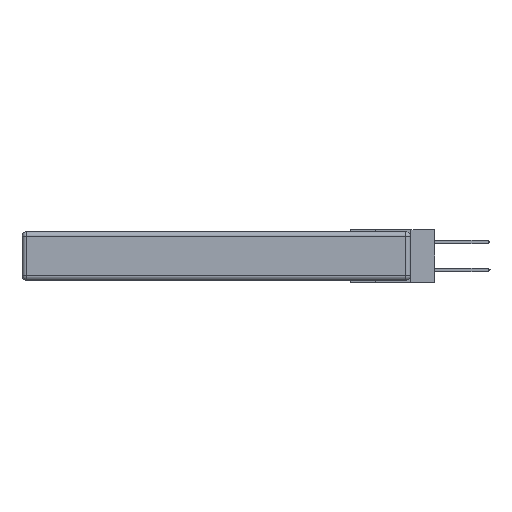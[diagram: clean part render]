
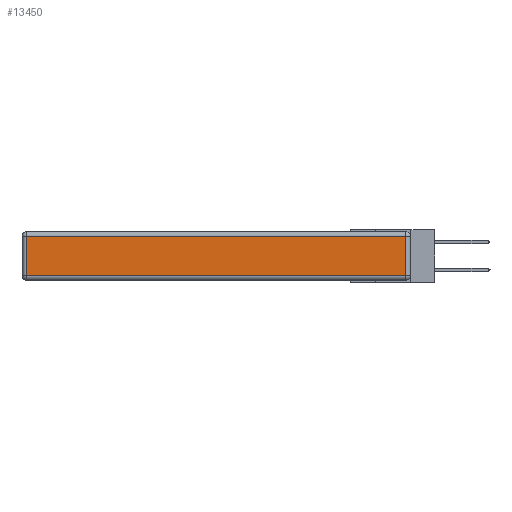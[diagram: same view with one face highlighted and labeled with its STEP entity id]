
A CAD part, left-side view. The second image highlights one B-rep face of the part: STEP entity #13450.
In plain terms, the highlighted planar face has unit normal (-1, 0, 0).
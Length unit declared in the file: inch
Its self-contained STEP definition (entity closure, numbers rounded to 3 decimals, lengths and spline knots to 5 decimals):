
#124 = CARTESIAN_POINT ( 'NONE',  ( 0., 0., -0.343 ) ) ;
#168 = DIRECTION ( 'NONE',  ( -1., 0., 0. ) ) ;
#174 = EDGE_CURVE ( 'NONE', #11928, #13129, #14936, .T. ) ;
#314 = EDGE_LOOP ( 'NONE', ( #872, #12004, #11875, #1644 ) ) ;
#712 = LINE ( 'NONE', #1514, #8168 ) ;
#872 = ORIENTED_EDGE ( 'NONE', *, *, #174, .T. ) ;
#1514 = CARTESIAN_POINT ( 'NONE',  ( 0., 2.75, -0.03 ) ) ;
#1644 = ORIENTED_EDGE ( 'NONE', *, *, #5004, .T. ) ;
#2084 = VERTEX_POINT ( 'NONE', #11034 ) ;
#4126 = AXIS2_PLACEMENT_3D ( 'NONE', #124, #168, #14631 ) ;
#4467 = CARTESIAN_POINT ( 'NONE',  ( 0., 2.72, -0.03 ) ) ;
#4505 = VERTEX_POINT ( 'NONE', #4467 ) ;
#5004 = EDGE_CURVE ( 'NONE', #4505, #11928, #15275, .T. ) ;
#5780 = LINE ( 'NONE', #14072, #13263 ) ;
#6287 = CARTESIAN_POINT ( 'NONE',  ( 0., 2.72, -0.313 ) ) ;
#6324 = EDGE_CURVE ( 'NONE', #13129, #2084, #5780, .T. ) ;
#6844 = VECTOR ( 'NONE', #8860, 39.37008 ) ;
#6981 = DIRECTION ( 'NONE',  ( 0., -1., 0. ) ) ;
#7283 = EDGE_CURVE ( 'NONE', #2084, #4505, #712, .T. ) ;
#8168 = VECTOR ( 'NONE', #11087, 39.37008 ) ;
#8237 = CARTESIAN_POINT ( 'NONE',  ( 0., 0., -0.313 ) ) ;
#8860 = DIRECTION ( 'NONE',  ( 0., 0., -1. ) ) ;
#9767 = PLANE ( 'NONE',  #4126 ) ;
#10147 = CARTESIAN_POINT ( 'NONE',  ( 0., 0.03, -0.313 ) ) ;
#11034 = CARTESIAN_POINT ( 'NONE',  ( 0., 0.03, -0.03 ) ) ;
#11087 = DIRECTION ( 'NONE',  ( 0., 1., 0. ) ) ;
#11250 = CARTESIAN_POINT ( 'NONE',  ( 0., 2.72, -0.343 ) ) ;
#11875 = ORIENTED_EDGE ( 'NONE', *, *, #7283, .T. ) ;
#11928 = VERTEX_POINT ( 'NONE', #6287 ) ;
#12004 = ORIENTED_EDGE ( 'NONE', *, *, #6324, .T. ) ;
#12034 = FACE_OUTER_BOUND ( 'NONE', #314, .T. ) ;
#13129 = VERTEX_POINT ( 'NONE', #10147 ) ;
#13263 = VECTOR ( 'NONE', #14020, 39.37008 ) ;
#13450 = ADVANCED_FACE ( 'NONE', ( #12034 ), #9767, .T. ) ;
#14020 = DIRECTION ( 'NONE',  ( 0., 0., 1. ) ) ;
#14072 = CARTESIAN_POINT ( 'NONE',  ( 0., 0.03, -0.343 ) ) ;
#14631 = DIRECTION ( 'NONE',  ( 0., 0., 1. ) ) ;
#14732 = VECTOR ( 'NONE', #6981, 39.37008 ) ;
#14936 = LINE ( 'NONE', #8237, #14732 ) ;
#15275 = LINE ( 'NONE', #11250, #6844 ) ;
